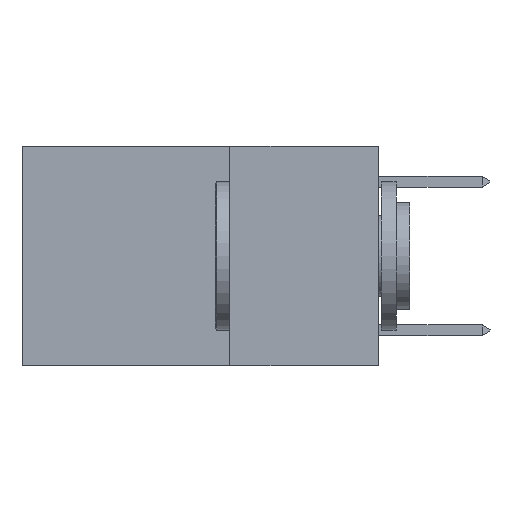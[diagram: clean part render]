
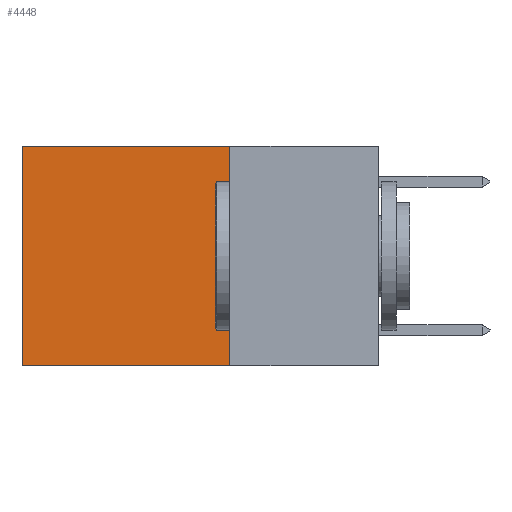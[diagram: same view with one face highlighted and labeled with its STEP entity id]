
A CAD part, left-side view. The second image highlights one B-rep face of the part: STEP entity #4448.
In plain terms, the highlighted planar face has unit normal (-1, 0, 0).
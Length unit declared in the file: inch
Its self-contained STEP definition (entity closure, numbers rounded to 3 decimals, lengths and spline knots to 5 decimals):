
#636 = LINE ( 'NONE', #5915, #6040 ) ;
#828 = DIRECTION ( 'NONE',  ( 0., 1., 0. ) ) ;
#1306 = EDGE_CURVE ( 'NONE', #9938, #11052, #636, .T. ) ;
#1513 = CARTESIAN_POINT ( 'NONE',  ( 0.2625, 0.6, -0.37 ) ) ;
#2397 = FACE_OUTER_BOUND ( 'NONE', #11652, .T. ) ;
#3519 = DIRECTION ( 'NONE',  ( 0., 1., 0. ) ) ;
#3807 = VERTEX_POINT ( 'NONE', #1513 ) ;
#3864 = CARTESIAN_POINT ( 'NONE',  ( 0.2625, 0.25, 0. ) ) ;
#4091 = CARTESIAN_POINT ( 'NONE',  ( 0.2625, 0.25, -0.37 ) ) ;
#4180 = LINE ( 'NONE', #4091, #9503 ) ;
#4448 = ADVANCED_FACE ( 'NONE', ( #2397 ), #5998, .F. ) ;
#5320 = DIRECTION ( 'NONE',  ( 0., 0., -1. ) ) ;
#5582 = EDGE_CURVE ( 'NONE', #11081, #3807, #10697, .T. ) ;
#5852 = CARTESIAN_POINT ( 'NONE',  ( 0.2625, 0.6, 0. ) ) ;
#5915 = CARTESIAN_POINT ( 'NONE',  ( 0.2625, 0.25, 0. ) ) ;
#5998 = PLANE ( 'NONE',  #12121 ) ;
#6040 = VECTOR ( 'NONE', #5320, 39.37008 ) ;
#6926 = ORIENTED_EDGE ( 'NONE', *, *, #5582, .T. ) ;
#7057 = ORIENTED_EDGE ( 'NONE', *, *, #13601, .F. ) ;
#7092 = DIRECTION ( 'NONE',  ( 0., 0., -1. ) ) ;
#7132 = ORIENTED_EDGE ( 'NONE', *, *, #1306, .F. ) ;
#7239 = ORIENTED_EDGE ( 'NONE', *, *, #9435, .T. ) ;
#7767 = CARTESIAN_POINT ( 'NONE',  ( 0.2625, 0.25, 0. ) ) ;
#7846 = CARTESIAN_POINT ( 'NONE',  ( 0.2625, 0.6, 0. ) ) ;
#7900 = VECTOR ( 'NONE', #10950, 39.37008 ) ;
#8394 = CARTESIAN_POINT ( 'NONE',  ( 0.2625, 0.25, 0. ) ) ;
#9019 = CARTESIAN_POINT ( 'NONE',  ( 0.2625, 0.25, -0.37 ) ) ;
#9435 = EDGE_CURVE ( 'NONE', #9938, #11081, #10754, .T. ) ;
#9503 = VECTOR ( 'NONE', #828, 39.37008 ) ;
#9938 = VERTEX_POINT ( 'NONE', #8394 ) ;
#10106 = VECTOR ( 'NONE', #3519, 39.37008 ) ;
#10697 = LINE ( 'NONE', #7846, #7900 ) ;
#10754 = LINE ( 'NONE', #7767, #10106 ) ;
#10950 = DIRECTION ( 'NONE',  ( 0., 0., -1. ) ) ;
#11052 = VERTEX_POINT ( 'NONE', #9019 ) ;
#11081 = VERTEX_POINT ( 'NONE', #5852 ) ;
#11652 = EDGE_LOOP ( 'NONE', ( #6926, #7057, #7132, #7239 ) ) ;
#12121 = AXIS2_PLACEMENT_3D ( 'NONE', #3864, #13264, #7092 ) ;
#13264 = DIRECTION ( 'NONE',  ( 1., 0., 0. ) ) ;
#13601 = EDGE_CURVE ( 'NONE', #11052, #3807, #4180, .T. ) ;
